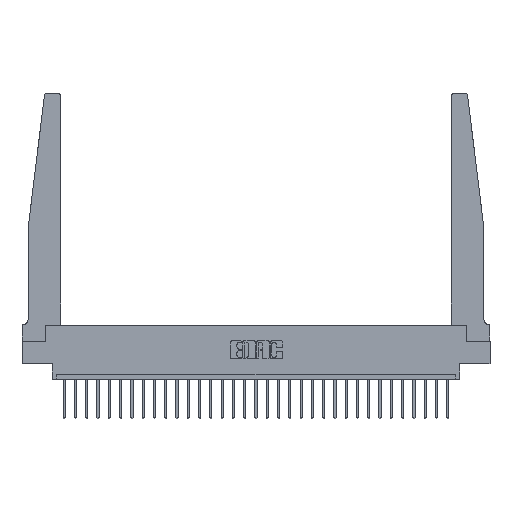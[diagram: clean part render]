
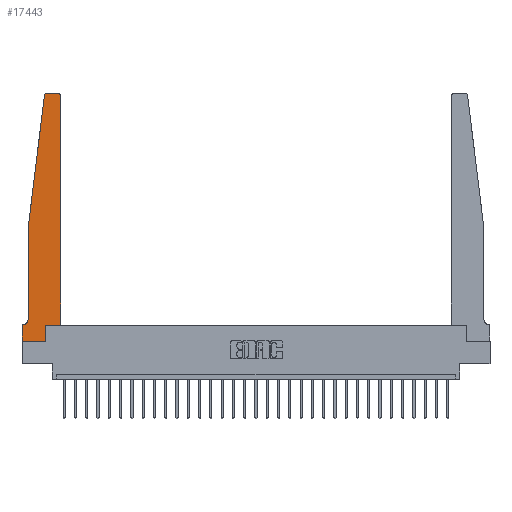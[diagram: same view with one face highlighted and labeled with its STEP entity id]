
A CAD part, top view. The second image highlights one B-rep face of the part: STEP entity #17443.
In plain terms, the highlighted planar face has unit normal (0, 0, 1).
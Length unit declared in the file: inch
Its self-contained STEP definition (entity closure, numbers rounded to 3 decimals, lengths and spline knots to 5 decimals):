
#91 = PLANE ( 'NONE',  #5976 ) ;
#338 = ORIENTED_EDGE ( 'NONE', *, *, #5090, .T. ) ;
#376 = LINE ( 'NONE', #9057, #1758 ) ;
#868 = DIRECTION ( 'NONE',  ( 1., 0., 0. ) ) ;
#1617 = VERTEX_POINT ( 'NONE', #20647 ) ;
#1655 = ORIENTED_EDGE ( 'NONE', *, *, #2119, .T. ) ;
#1686 = CARTESIAN_POINT ( 'NONE',  ( 0.395, 2.72, 0.37 ) ) ;
#1758 = VECTOR ( 'NONE', #17653, 39.37008 ) ;
#2119 = EDGE_CURVE ( 'NONE', #13105, #4995, #25849, .T. ) ;
#2180 = VECTOR ( 'NONE', #6635, 39.37008 ) ;
#2851 = CIRCLE ( 'NONE', #25933, 0.03 ) ;
#3436 = VECTOR ( 'NONE', #24029, 39.37008 ) ;
#3956 = CARTESIAN_POINT ( 'NONE',  ( 0., 0.1875, 0.37 ) ) ;
#4488 = DIRECTION ( 'NONE',  ( 0., 0., 1. ) ) ;
#4691 = LINE ( 'NONE', #4823, #5889 ) ;
#4823 = CARTESIAN_POINT ( 'NONE',  ( 0., 0., 0.37 ) ) ;
#4865 = EDGE_CURVE ( 'NONE', #24066, #23043, #23920, .T. ) ;
#4995 = VERTEX_POINT ( 'NONE', #21381 ) ;
#5090 = EDGE_CURVE ( 'NONE', #14642, #8169, #376, .T. ) ;
#5165 = LINE ( 'NONE', #26288, #3436 ) ;
#5457 = EDGE_CURVE ( 'NONE', #24507, #25637, #5165, .T. ) ;
#5467 = VECTOR ( 'NONE', #7363, 39.37008 ) ;
#5570 = CIRCLE ( 'NONE', #14154, 0.05 ) ;
#5884 = DIRECTION ( 'NONE',  ( 0., 1., 0. ) ) ;
#5889 = VECTOR ( 'NONE', #23962, 39.37008 ) ;
#5931 = EDGE_LOOP ( 'NONE', ( #23905, #17442, #12529, #8415, #23481, #5966, #6507, #15262, #338, #16924, #1655, #10277 ) ) ;
#5941 = CARTESIAN_POINT ( 'NONE',  ( 0., 0., 0.37 ) ) ;
#5966 = ORIENTED_EDGE ( 'NONE', *, *, #5457, .T. ) ;
#5972 = EDGE_CURVE ( 'NONE', #7414, #14642, #27085, .T. ) ;
#5976 = AXIS2_PLACEMENT_3D ( 'NONE', #8762, #4488, #15232 ) ;
#6181 = EDGE_CURVE ( 'NONE', #4995, #24066, #14479, .T. ) ;
#6288 = VERTEX_POINT ( 'NONE', #13191 ) ;
#6304 = EDGE_CURVE ( 'NONE', #25637, #7414, #4691, .T. ) ;
#6507 = ORIENTED_EDGE ( 'NONE', *, *, #6304, .T. ) ;
#6635 = DIRECTION ( 'NONE',  ( -1., 0., 0. ) ) ;
#7363 = DIRECTION ( 'NONE',  ( -0.122, -0.992, 0. ) ) ;
#7414 = VERTEX_POINT ( 'NONE', #5941 ) ;
#7437 = DIRECTION ( 'NONE',  ( 0., 0., -1. ) ) ;
#7975 = LINE ( 'NONE', #16588, #21917 ) ;
#8169 = VERTEX_POINT ( 'NONE', #20997 ) ;
#8415 = ORIENTED_EDGE ( 'NONE', *, *, #26787, .T. ) ;
#8762 = CARTESIAN_POINT ( 'NONE',  ( 0., 0.1875, 0.37 ) ) ;
#9057 = CARTESIAN_POINT ( 'NONE',  ( 0.2605, 0.18, 0.37 ) ) ;
#9203 = CARTESIAN_POINT ( 'NONE',  ( 0.065, 0.2375, 0.37 ) ) ;
#10243 = DIRECTION ( 'NONE',  ( 0., 0., 1. ) ) ;
#10277 = ORIENTED_EDGE ( 'NONE', *, *, #6181, .T. ) ;
#10485 = CARTESIAN_POINT ( 'NONE',  ( 0.25, 2.75, 0.37 ) ) ;
#10649 = DIRECTION ( 'NONE',  ( 0., -1., 0. ) ) ;
#10889 = VECTOR ( 'NONE', #10649, 39.37008 ) ;
#11552 = DIRECTION ( 'NONE',  ( -1., 0., 0. ) ) ;
#12262 = AXIS2_PLACEMENT_3D ( 'NONE', #1686, #10243, #12646 ) ;
#12529 = ORIENTED_EDGE ( 'NONE', *, *, #15810, .T. ) ;
#12646 = DIRECTION ( 'NONE',  ( 1., 0., 0. ) ) ;
#13105 = VERTEX_POINT ( 'NONE', #18349 ) ;
#13191 = CARTESIAN_POINT ( 'NONE',  ( 0.065, 1.25, 0.37 ) ) ;
#13760 = CARTESIAN_POINT ( 'NONE',  ( 0., 0., 0.37 ) ) ;
#13841 = CARTESIAN_POINT ( 'NONE',  ( 0.065, 1.25, 0.37 ) ) ;
#14154 = AXIS2_PLACEMENT_3D ( 'NONE', #24287, #7437, #11552 ) ;
#14479 = CIRCLE ( 'NONE', #12262, 0.03 ) ;
#14642 = VERTEX_POINT ( 'NONE', #15816 ) ;
#15232 = DIRECTION ( 'NONE',  ( 1., 0., 0. ) ) ;
#15262 = ORIENTED_EDGE ( 'NONE', *, *, #5972, .T. ) ;
#15810 = EDGE_CURVE ( 'NONE', #1617, #6288, #19953, .T. ) ;
#15816 = CARTESIAN_POINT ( 'NONE',  ( 0.2605, 0., 0.37 ) ) ;
#16086 = CARTESIAN_POINT ( 'NONE',  ( 0.27653, 2.75, 0.37 ) ) ;
#16588 = CARTESIAN_POINT ( 'NONE',  ( 0.425, 0.18, 0.37 ) ) ;
#16635 = CARTESIAN_POINT ( 'NONE',  ( 0.425, 0.18, 0.37 ) ) ;
#16924 = ORIENTED_EDGE ( 'NONE', *, *, #19681, .T. ) ;
#17142 = CARTESIAN_POINT ( 'NONE',  ( 0.395, 2.75, 0.37 ) ) ;
#17442 = ORIENTED_EDGE ( 'NONE', *, *, #18325, .T. ) ;
#17443 = ADVANCED_FACE ( 'NONE', ( #26159 ), #91, .T. ) ;
#17653 = DIRECTION ( 'NONE',  ( 0., 1., 0. ) ) ;
#17985 = EDGE_CURVE ( 'NONE', #27461, #24507, #5570, .T. ) ;
#18325 = EDGE_CURVE ( 'NONE', #23043, #1617, #2851, .T. ) ;
#18349 = CARTESIAN_POINT ( 'NONE',  ( 0.425, 0.18, 0.37 ) ) ;
#19676 = CARTESIAN_POINT ( 'NONE',  ( 0.065, 1.25, 0.37 ) ) ;
#19681 = EDGE_CURVE ( 'NONE', #8169, #13105, #7975, .T. ) ;
#19855 = DIRECTION ( 'NONE',  ( 0., 0., 1. ) ) ;
#19953 = LINE ( 'NONE', #13841, #5467 ) ;
#20647 = CARTESIAN_POINT ( 'NONE',  ( 0.24675, 2.72367, 0.37 ) ) ;
#20699 = LINE ( 'NONE', #19676, #10889 ) ;
#20816 = VECTOR ( 'NONE', #22564, 39.37008 ) ;
#20997 = CARTESIAN_POINT ( 'NONE',  ( 0.2605, 0.18, 0.37 ) ) ;
#21381 = CARTESIAN_POINT ( 'NONE',  ( 0.425, 2.72, 0.37 ) ) ;
#21768 = CARTESIAN_POINT ( 'NONE',  ( 0.015, 0.1875, 0.37 ) ) ;
#21917 = VECTOR ( 'NONE', #868, 39.37008 ) ;
#22564 = DIRECTION ( 'NONE',  ( 1., 0., 0. ) ) ;
#23043 = VERTEX_POINT ( 'NONE', #16086 ) ;
#23481 = ORIENTED_EDGE ( 'NONE', *, *, #17985, .T. ) ;
#23905 = ORIENTED_EDGE ( 'NONE', *, *, #4865, .T. ) ;
#23920 = LINE ( 'NONE', #10485, #2180 ) ;
#23962 = DIRECTION ( 'NONE',  ( 0., -1., 0. ) ) ;
#24029 = DIRECTION ( 'NONE',  ( -1., 0., 0. ) ) ;
#24066 = VERTEX_POINT ( 'NONE', #17142 ) ;
#24287 = CARTESIAN_POINT ( 'NONE',  ( 0.015, 0.2375, 0.37 ) ) ;
#24507 = VERTEX_POINT ( 'NONE', #21768 ) ;
#25637 = VERTEX_POINT ( 'NONE', #3956 ) ;
#25849 = LINE ( 'NONE', #16635, #25857 ) ;
#25857 = VECTOR ( 'NONE', #5884, 39.37008 ) ;
#25933 = AXIS2_PLACEMENT_3D ( 'NONE', #26387, #19855, #26520 ) ;
#26159 = FACE_OUTER_BOUND ( 'NONE', #5931, .T. ) ;
#26288 = CARTESIAN_POINT ( 'NONE',  ( 0.065, 0.1875, 0.37 ) ) ;
#26387 = CARTESIAN_POINT ( 'NONE',  ( 0.27653, 2.72, 0.37 ) ) ;
#26520 = DIRECTION ( 'NONE',  ( 1., 0., 0. ) ) ;
#26787 = EDGE_CURVE ( 'NONE', #6288, #27461, #20699, .T. ) ;
#27085 = LINE ( 'NONE', #13760, #20816 ) ;
#27461 = VERTEX_POINT ( 'NONE', #9203 ) ;
